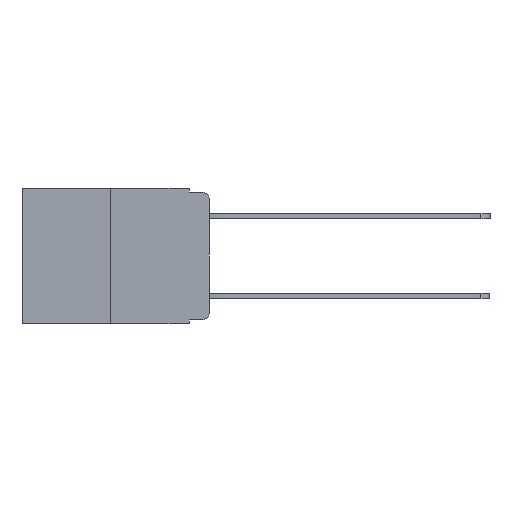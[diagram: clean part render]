
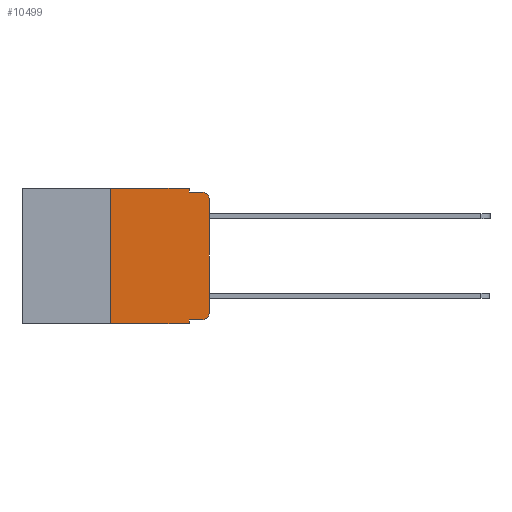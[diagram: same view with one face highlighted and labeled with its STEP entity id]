
A CAD part, left-side view. The second image highlights one B-rep face of the part: STEP entity #10499.
In plain terms, the highlighted planar face has unit normal (-1, 0, 0).
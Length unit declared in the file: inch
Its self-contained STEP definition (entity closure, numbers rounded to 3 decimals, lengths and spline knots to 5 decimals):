
#1583 = FACE_OUTER_BOUND ( 'NONE', #9693, .T. ) ;
#1606 = CIRCLE ( 'NONE', #23035, 0.02 ) ;
#1777 = ORIENTED_EDGE ( 'NONE', *, *, #14511, .T. ) ;
#1949 = CARTESIAN_POINT ( 'NONE',  ( 0., 0.02, -0.03 ) ) ;
#2341 = VERTEX_POINT ( 'NONE', #9568 ) ;
#2447 = CARTESIAN_POINT ( 'NONE',  ( 0., 0.02, -0.01 ) ) ;
#2997 = CARTESIAN_POINT ( 'NONE',  ( 0., 0.051, 0. ) ) ;
#3003 = LINE ( 'NONE', #24660, #12647 ) ;
#3369 = CARTESIAN_POINT ( 'NONE',  ( 0., 0.051, -0.343 ) ) ;
#3429 = CARTESIAN_POINT ( 'NONE',  ( 0., 0.051, 0. ) ) ;
#4279 = ORIENTED_EDGE ( 'NONE', *, *, #13801, .F. ) ;
#4381 = EDGE_CURVE ( 'NONE', #16971, #23046, #22755, .T. ) ;
#4407 = ORIENTED_EDGE ( 'NONE', *, *, #9629, .F. ) ;
#4745 = EDGE_CURVE ( 'NONE', #2341, #5706, #11673, .T. ) ;
#5007 = LINE ( 'NONE', #20360, #14587 ) ;
#5368 = DIRECTION ( 'NONE',  ( 0., 0., -1. ) ) ;
#5651 = CARTESIAN_POINT ( 'NONE',  ( 0., 0.25, 0. ) ) ;
#5706 = VERTEX_POINT ( 'NONE', #2447 ) ;
#6160 = CARTESIAN_POINT ( 'NONE',  ( 0., 0.473, 0. ) ) ;
#6503 = CARTESIAN_POINT ( 'NONE',  ( 0., 0.051, -0.01 ) ) ;
#6585 = VERTEX_POINT ( 'NONE', #3369 ) ;
#6620 = DIRECTION ( 'NONE',  ( -1., 0., 0. ) ) ;
#6654 = LINE ( 'NONE', #21210, #21112 ) ;
#7063 = CARTESIAN_POINT ( 'NONE',  ( 0., 0.25, -0.343 ) ) ;
#7190 = ORIENTED_EDGE ( 'NONE', *, *, #13418, .F. ) ;
#7204 = CARTESIAN_POINT ( 'NONE',  ( 0., 0., -0.313 ) ) ;
#7237 = VERTEX_POINT ( 'NONE', #7063 ) ;
#7713 = VERTEX_POINT ( 'NONE', #6503 ) ;
#7733 = VECTOR ( 'NONE', #20585, 39.37008 ) ;
#8092 = DIRECTION ( 'NONE',  ( 0., 0., 1. ) ) ;
#8141 = DIRECTION ( 'NONE',  ( 0., -1., 0. ) ) ;
#8537 = VECTOR ( 'NONE', #23926, 39.37008 ) ;
#9018 = CARTESIAN_POINT ( 'NONE',  ( 0., 0.051, -0.333 ) ) ;
#9103 = VERTEX_POINT ( 'NONE', #7204 ) ;
#9568 = CARTESIAN_POINT ( 'NONE',  ( 0., 0., -0.03 ) ) ;
#9603 = DIRECTION ( 'NONE',  ( 0., 0., -1. ) ) ;
#9629 = EDGE_CURVE ( 'NONE', #16971, #6585, #19467, .T. ) ;
#9693 = EDGE_LOOP ( 'NONE', ( #20308, #12298, #10541, #22373, #4279, #7190, #1777, #4407, #15411, #20208 ) ) ;
#9998 = CARTESIAN_POINT ( 'NONE',  ( 0., 0.051, -0.333 ) ) ;
#10499 = ADVANCED_FACE ( 'NONE', ( #1583 ), #17050, .F. ) ;
#10541 = ORIENTED_EDGE ( 'NONE', *, *, #23421, .F. ) ;
#10850 = CARTESIAN_POINT ( 'NONE',  ( 0., 0.25, 0. ) ) ;
#11673 = CIRCLE ( 'NONE', #16940, 0.02 ) ;
#11840 = VERTEX_POINT ( 'NONE', #5651 ) ;
#11963 = LINE ( 'NONE', #3429, #21260 ) ;
#12298 = ORIENTED_EDGE ( 'NONE', *, *, #4745, .T. ) ;
#12647 = VECTOR ( 'NONE', #19087, 39.37008 ) ;
#13314 = CARTESIAN_POINT ( 'NONE',  ( 0., 0.473, 0. ) ) ;
#13418 = EDGE_CURVE ( 'NONE', #7237, #11840, #19125, .T. ) ;
#13561 = LINE ( 'NONE', #6160, #22926 ) ;
#13801 = EDGE_CURVE ( 'NONE', #11840, #16080, #13561, .T. ) ;
#13911 = EDGE_CURVE ( 'NONE', #9103, #2341, #6654, .T. ) ;
#14511 = EDGE_CURVE ( 'NONE', #7237, #6585, #3003, .T. ) ;
#14587 = VECTOR ( 'NONE', #22255, 39.37008 ) ;
#15128 = VECTOR ( 'NONE', #20006, 39.37008 ) ;
#15411 = ORIENTED_EDGE ( 'NONE', *, *, #4381, .T. ) ;
#15922 = AXIS2_PLACEMENT_3D ( 'NONE', #13314, #20782, #9603 ) ;
#16080 = VERTEX_POINT ( 'NONE', #21900 ) ;
#16940 = AXIS2_PLACEMENT_3D ( 'NONE', #1949, #18896, #18865 ) ;
#16971 = VERTEX_POINT ( 'NONE', #9998 ) ;
#17050 = PLANE ( 'NONE',  #15922 ) ;
#17987 = CARTESIAN_POINT ( 'NONE',  ( 0., 0.02, -0.313 ) ) ;
#18865 = DIRECTION ( 'NONE',  ( 0., 0., -1. ) ) ;
#18896 = DIRECTION ( 'NONE',  ( -1., 0., 0. ) ) ;
#19087 = DIRECTION ( 'NONE',  ( 0., -1., 0. ) ) ;
#19125 = LINE ( 'NONE', #10850, #8537 ) ;
#19467 = LINE ( 'NONE', #2997, #15128 ) ;
#19624 = EDGE_CURVE ( 'NONE', #16080, #7713, #11963, .T. ) ;
#19840 = DIRECTION ( 'NONE',  ( 0., 0., -1. ) ) ;
#20006 = DIRECTION ( 'NONE',  ( 0., 0., -1. ) ) ;
#20208 = ORIENTED_EDGE ( 'NONE', *, *, #23884, .T. ) ;
#20308 = ORIENTED_EDGE ( 'NONE', *, *, #13911, .T. ) ;
#20360 = CARTESIAN_POINT ( 'NONE',  ( 0., 0.051, -0.01 ) ) ;
#20585 = DIRECTION ( 'NONE',  ( 0., -1., 0. ) ) ;
#20782 = DIRECTION ( 'NONE',  ( 1., 0., 0. ) ) ;
#21112 = VECTOR ( 'NONE', #8092, 39.37008 ) ;
#21210 = CARTESIAN_POINT ( 'NONE',  ( 0., 0., 0. ) ) ;
#21260 = VECTOR ( 'NONE', #5368, 39.37008 ) ;
#21900 = CARTESIAN_POINT ( 'NONE',  ( 0., 0.051, 0. ) ) ;
#22255 = DIRECTION ( 'NONE',  ( 0., -1., 0. ) ) ;
#22373 = ORIENTED_EDGE ( 'NONE', *, *, #19624, .F. ) ;
#22755 = LINE ( 'NONE', #9018, #7733 ) ;
#22926 = VECTOR ( 'NONE', #8141, 39.37008 ) ;
#23035 = AXIS2_PLACEMENT_3D ( 'NONE', #17987, #6620, #19840 ) ;
#23046 = VERTEX_POINT ( 'NONE', #23181 ) ;
#23181 = CARTESIAN_POINT ( 'NONE',  ( 0., 0.02, -0.333 ) ) ;
#23421 = EDGE_CURVE ( 'NONE', #7713, #5706, #5007, .T. ) ;
#23884 = EDGE_CURVE ( 'NONE', #23046, #9103, #1606, .T. ) ;
#23926 = DIRECTION ( 'NONE',  ( 0., 0., 1. ) ) ;
#24660 = CARTESIAN_POINT ( 'NONE',  ( 0., 0.473, -0.343 ) ) ;
